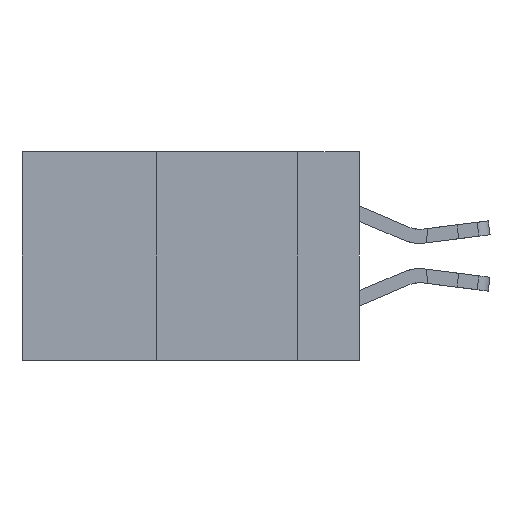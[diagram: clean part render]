
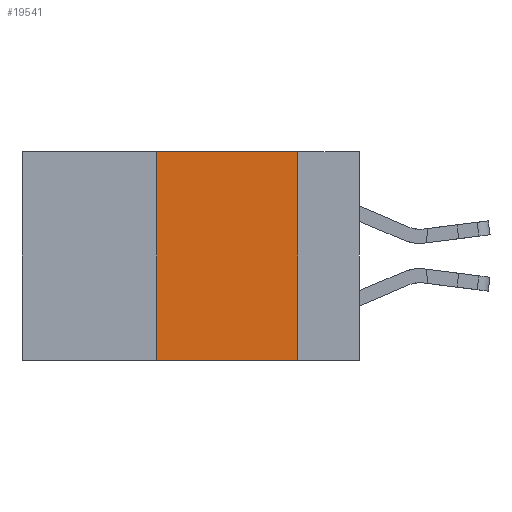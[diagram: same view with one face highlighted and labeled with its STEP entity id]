
A CAD part, left-side view. The second image highlights one B-rep face of the part: STEP entity #19541.
In plain terms, the highlighted planar face has unit normal (-1, 0, 0).
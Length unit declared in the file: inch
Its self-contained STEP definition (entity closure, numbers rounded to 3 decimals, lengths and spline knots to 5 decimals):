
#423 = VERTEX_POINT ( 'NONE', #7254 ) ;
#1034 = VERTEX_POINT ( 'NONE', #14369 ) ;
#1794 = LINE ( 'NONE', #12889, #10195 ) ;
#2065 = LINE ( 'NONE', #7191, #5258 ) ;
#2584 = CARTESIAN_POINT ( 'NONE',  ( 0., 0.6, -0.37 ) ) ;
#4993 = DIRECTION ( 'NONE',  ( 0., -1., 0. ) ) ;
#5258 = VECTOR ( 'NONE', #19841, 39.37008 ) ;
#5350 = CARTESIAN_POINT ( 'NONE',  ( 0., 0.6, 0. ) ) ;
#5596 = VERTEX_POINT ( 'NONE', #13741 ) ;
#7174 = PLANE ( 'NONE',  #12576 ) ;
#7191 = CARTESIAN_POINT ( 'NONE',  ( 0., 0.36, 0. ) ) ;
#7215 = VECTOR ( 'NONE', #11657, 39.37008 ) ;
#7254 = CARTESIAN_POINT ( 'NONE',  ( 0., 0.36, -0.37 ) ) ;
#8573 = ORIENTED_EDGE ( 'NONE', *, *, #9137, .F. ) ;
#9137 = EDGE_CURVE ( 'NONE', #423, #5596, #2065, .T. ) ;
#10195 = VECTOR ( 'NONE', #4993, 39.37008 ) ;
#10315 = DIRECTION ( 'NONE',  ( 1., 0., 0. ) ) ;
#10554 = EDGE_CURVE ( 'NONE', #1034, #15885, #11384, .T. ) ;
#11384 = LINE ( 'NONE', #11731, #7215 ) ;
#11657 = DIRECTION ( 'NONE',  ( 0., 0., -1. ) ) ;
#11731 = CARTESIAN_POINT ( 'NONE',  ( 0., 0.11, 0. ) ) ;
#12576 = AXIS2_PLACEMENT_3D ( 'NONE', #5350, #10315, #18015 ) ;
#12889 = CARTESIAN_POINT ( 'NONE',  ( 0., 0.6, 0. ) ) ;
#13552 = DIRECTION ( 'NONE',  ( 0., -1., 0. ) ) ;
#13561 = EDGE_CURVE ( 'NONE', #5596, #1034, #1794, .T. ) ;
#13741 = CARTESIAN_POINT ( 'NONE',  ( 0., 0.36, 0. ) ) ;
#14369 = CARTESIAN_POINT ( 'NONE',  ( 0., 0.11, 0. ) ) ;
#14399 = ORIENTED_EDGE ( 'NONE', *, *, #10554, .F. ) ;
#14529 = EDGE_LOOP ( 'NONE', ( #14399, #16164, #8573, #15933 ) ) ;
#14947 = FACE_OUTER_BOUND ( 'NONE', #14529, .T. ) ;
#15885 = VERTEX_POINT ( 'NONE', #16235 ) ;
#15933 = ORIENTED_EDGE ( 'NONE', *, *, #20289, .T. ) ;
#16164 = ORIENTED_EDGE ( 'NONE', *, *, #13561, .F. ) ;
#16235 = CARTESIAN_POINT ( 'NONE',  ( 0., 0.11, -0.37 ) ) ;
#16779 = LINE ( 'NONE', #2584, #19214 ) ;
#18015 = DIRECTION ( 'NONE',  ( 0., 0., -1. ) ) ;
#19214 = VECTOR ( 'NONE', #13552, 39.37008 ) ;
#19541 = ADVANCED_FACE ( 'NONE', ( #14947 ), #7174, .F. ) ;
#19841 = DIRECTION ( 'NONE',  ( 0., 0., 1. ) ) ;
#20289 = EDGE_CURVE ( 'NONE', #423, #15885, #16779, .T. ) ;
